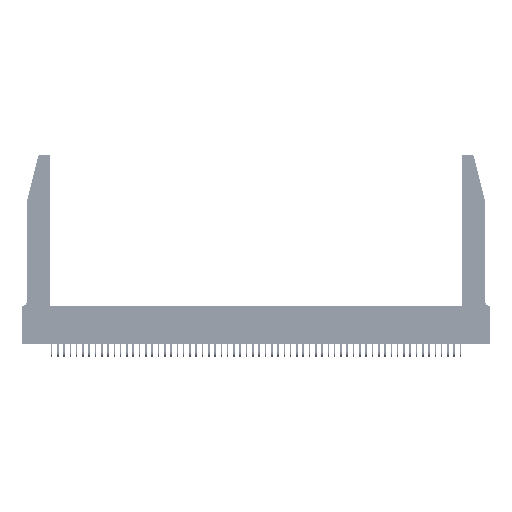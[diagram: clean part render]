
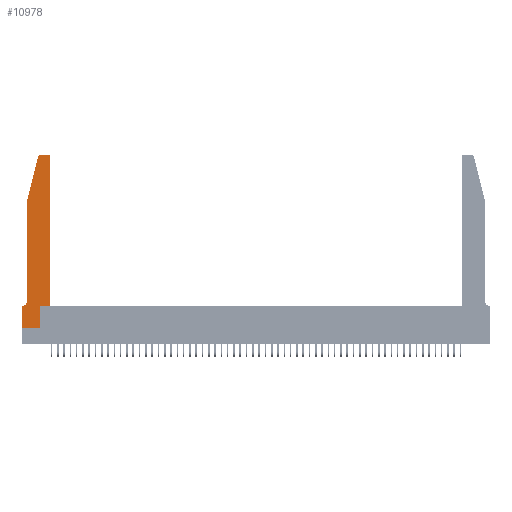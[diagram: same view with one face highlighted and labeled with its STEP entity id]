
A CAD part, top view. The second image highlights one B-rep face of the part: STEP entity #10978.
In plain terms, the highlighted planar face has unit normal (0, 0, 1).
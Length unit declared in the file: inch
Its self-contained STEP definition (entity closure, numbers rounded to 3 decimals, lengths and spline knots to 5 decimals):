
#1144 = EDGE_CURVE ( 'NONE', #27276, #46740, #19152, .T. ) ;
#1185 = ORIENTED_EDGE ( 'NONE', *, *, #3137, .T. ) ;
#1265 = CARTESIAN_POINT ( 'NONE',  ( 0.4505, 0.35, 0.37 ) ) ;
#1358 = ORIENTED_EDGE ( 'NONE', *, *, #42445, .T. ) ;
#1390 = VECTOR ( 'NONE', #35444, 39.37008 ) ;
#2430 = ORIENTED_EDGE ( 'NONE', *, *, #13091, .T. ) ;
#2660 = EDGE_CURVE ( 'NONE', #15259, #50603, #51960, .T. ) ;
#2677 = ORIENTED_EDGE ( 'NONE', *, *, #2660, .T. ) ;
#2962 = CARTESIAN_POINT ( 'NONE',  ( 0.2605, 2.75, 0.37 ) ) ;
#3137 = EDGE_CURVE ( 'NONE', #53790, #24854, #18341, .T. ) ;
#3493 = AXIS2_PLACEMENT_3D ( 'NONE', #33217, #7725, #37428 ) ;
#3852 = VERTEX_POINT ( 'NONE', #5821 ) ;
#4472 = LINE ( 'NONE', #11216, #25912 ) ;
#5068 = CARTESIAN_POINT ( 'NONE',  ( 0.0755, 0.42, 0.37 ) ) ;
#5821 = CARTESIAN_POINT ( 'NONE',  ( 0.4205, 2.75, 0.37 ) ) ;
#5848 = DIRECTION ( 'NONE',  ( 0., 0., 1. ) ) ;
#5897 = ORIENTED_EDGE ( 'NONE', *, *, #17350, .T. ) ;
#6249 = CARTESIAN_POINT ( 'NONE',  ( 0.4505, 2.72, 0.37 ) ) ;
#6460 = CARTESIAN_POINT ( 'NONE',  ( 0., 0., 0.37 ) ) ;
#6992 = ORIENTED_EDGE ( 'NONE', *, *, #1144, .T. ) ;
#7110 = AXIS2_PLACEMENT_3D ( 'NONE', #21053, #42389, #17166 ) ;
#7152 = LINE ( 'NONE', #9784, #39676 ) ;
#7649 = ORIENTED_EDGE ( 'NONE', *, *, #35547, .T. ) ;
#7725 = DIRECTION ( 'NONE',  ( 0., 0., 1. ) ) ;
#9075 = VECTOR ( 'NONE', #31203, 39.37008 ) ;
#9408 = VECTOR ( 'NONE', #23684, 39.37008 ) ;
#9784 = CARTESIAN_POINT ( 'NONE',  ( 0.2865, 0.35, 0.37 ) ) ;
#10311 = ORIENTED_EDGE ( 'NONE', *, *, #40543, .T. ) ;
#10978 = ADVANCED_FACE ( 'NONE', ( #45802 ), #33964, .T. ) ;
#11152 = DIRECTION ( 'NONE',  ( -0.239, -0.971, 0. ) ) ;
#11216 = CARTESIAN_POINT ( 'NONE',  ( 0.4505, 0.35, 0.37 ) ) ;
#11679 = ORIENTED_EDGE ( 'NONE', *, *, #34342, .T. ) ;
#11734 = CARTESIAN_POINT ( 'NONE',  ( 0.4505, 0.35, 0.37 ) ) ;
#11985 = CARTESIAN_POINT ( 'NONE',  ( 0.0755, 2., 0.37 ) ) ;
#12399 = LINE ( 'NONE', #2962, #32286 ) ;
#13091 = EDGE_CURVE ( 'NONE', #15248, #53790, #17243, .T. ) ;
#13307 = AXIS2_PLACEMENT_3D ( 'NONE', #31402, #5848, #35607 ) ;
#13416 = EDGE_CURVE ( 'NONE', #46740, #3852, #35022, .T. ) ;
#13746 = EDGE_CURVE ( 'NONE', #28227, #54357, #7152, .T. ) ;
#14112 = DIRECTION ( 'NONE',  ( 0., 1., 0. ) ) ;
#14314 = VECTOR ( 'NONE', #23885, 39.37008 ) ;
#14790 = CARTESIAN_POINT ( 'NONE',  ( 0., 0., 0.37 ) ) ;
#15248 = VERTEX_POINT ( 'NONE', #41295 ) ;
#15259 = VERTEX_POINT ( 'NONE', #28797 ) ;
#16382 = ORIENTED_EDGE ( 'NONE', *, *, #13416, .T. ) ;
#17166 = DIRECTION ( 'NONE',  ( 1., 0., 0. ) ) ;
#17221 = ORIENTED_EDGE ( 'NONE', *, *, #13746, .T. ) ;
#17243 = CIRCLE ( 'NONE', #13307, 0.03 ) ;
#17350 = EDGE_CURVE ( 'NONE', #37437, #15259, #20083, .T. ) ;
#18341 = LINE ( 'NONE', #36526, #29586 ) ;
#18676 = CARTESIAN_POINT ( 'NONE',  ( 0., 0., 0.37 ) ) ;
#19152 = LINE ( 'NONE', #1265, #9075 ) ;
#20083 = CIRCLE ( 'NONE', #52610, 0.07 ) ;
#20294 = LINE ( 'NONE', #18676, #1390 ) ;
#20798 = LINE ( 'NONE', #6460, #9408 ) ;
#20909 = CARTESIAN_POINT ( 'NONE',  ( 0.0755, 0.35, 0.37 ) ) ;
#21053 = CARTESIAN_POINT ( 'NONE',  ( 0., 0.35, 0.37 ) ) ;
#21184 = EDGE_CURVE ( 'NONE', #50603, #50009, #20294, .T. ) ;
#21426 = CARTESIAN_POINT ( 'NONE',  ( 0.0055, 0.42, 0.37 ) ) ;
#23684 = DIRECTION ( 'NONE',  ( 1., 0., 0. ) ) ;
#23885 = DIRECTION ( 'NONE',  ( 0., -1., 0. ) ) ;
#24854 = VERTEX_POINT ( 'NONE', #11985 ) ;
#25166 = DIRECTION ( 'NONE',  ( -1., 0., 0. ) ) ;
#25652 = DIRECTION ( 'NONE',  ( -1., 0., 0. ) ) ;
#25912 = VECTOR ( 'NONE', #49040, 39.37008 ) ;
#27276 = VERTEX_POINT ( 'NONE', #11734 ) ;
#28227 = VERTEX_POINT ( 'NONE', #29233 ) ;
#28797 = CARTESIAN_POINT ( 'NONE',  ( 0.0055, 0.35, 0.37 ) ) ;
#29233 = CARTESIAN_POINT ( 'NONE',  ( 0.2865, 0., 0.37 ) ) ;
#29586 = VECTOR ( 'NONE', #11152, 39.37008 ) ;
#31203 = DIRECTION ( 'NONE',  ( 0., 1., 0. ) ) ;
#31402 = CARTESIAN_POINT ( 'NONE',  ( 0.284, 2.72, 0.37 ) ) ;
#32286 = VECTOR ( 'NONE', #41272, 39.37008 ) ;
#33217 = CARTESIAN_POINT ( 'NONE',  ( 0.4205, 2.72, 0.37 ) ) ;
#33379 = CARTESIAN_POINT ( 'NONE',  ( 0.25487, 2.72718, 0.37 ) ) ;
#33964 = PLANE ( 'NONE',  #7110 ) ;
#34342 = EDGE_CURVE ( 'NONE', #3852, #15248, #12399, .T. ) ;
#35022 = CIRCLE ( 'NONE', #3493, 0.03 ) ;
#35198 = ORIENTED_EDGE ( 'NONE', *, *, #21184, .T. ) ;
#35444 = DIRECTION ( 'NONE',  ( 0., -1., 0. ) ) ;
#35547 = EDGE_CURVE ( 'NONE', #54357, #27276, #4472, .T. ) ;
#35607 = DIRECTION ( 'NONE',  ( 1., 0., 0. ) ) ;
#36526 = CARTESIAN_POINT ( 'NONE',  ( 0.0755, 2., 0.37 ) ) ;
#36805 = LINE ( 'NONE', #40624, #14314 ) ;
#37428 = DIRECTION ( 'NONE',  ( 1., 0., 0. ) ) ;
#37437 = VERTEX_POINT ( 'NONE', #5068 ) ;
#39676 = VECTOR ( 'NONE', #14112, 39.37008 ) ;
#40543 = EDGE_CURVE ( 'NONE', #50009, #28227, #20798, .T. ) ;
#40624 = CARTESIAN_POINT ( 'NONE',  ( 0.0755, 2., 0.37 ) ) ;
#41272 = DIRECTION ( 'NONE',  ( -1., 0., 0. ) ) ;
#41295 = CARTESIAN_POINT ( 'NONE',  ( 0.284, 2.75, 0.37 ) ) ;
#42389 = DIRECTION ( 'NONE',  ( 0., 0., 1. ) ) ;
#42445 = EDGE_CURVE ( 'NONE', #24854, #37437, #36805, .T. ) ;
#45802 = FACE_OUTER_BOUND ( 'NONE', #51962, .T. ) ;
#46740 = VERTEX_POINT ( 'NONE', #6249 ) ;
#49040 = DIRECTION ( 'NONE',  ( 1., 0., 0. ) ) ;
#49807 = CARTESIAN_POINT ( 'NONE',  ( 0.2865, 0.35, 0.37 ) ) ;
#50009 = VERTEX_POINT ( 'NONE', #14790 ) ;
#50603 = VERTEX_POINT ( 'NONE', #52294 ) ;
#50617 = VECTOR ( 'NONE', #25166, 39.37008 ) ;
#50803 = DIRECTION ( 'NONE',  ( 0., 0., -1. ) ) ;
#51960 = LINE ( 'NONE', #20909, #50617 ) ;
#51962 = EDGE_LOOP ( 'NONE', ( #11679, #2430, #1185, #1358, #5897, #2677, #35198, #10311, #17221, #7649, #6992, #16382 ) ) ;
#52294 = CARTESIAN_POINT ( 'NONE',  ( 0., 0.35, 0.37 ) ) ;
#52610 = AXIS2_PLACEMENT_3D ( 'NONE', #21426, #50803, #25652 ) ;
#53790 = VERTEX_POINT ( 'NONE', #33379 ) ;
#54357 = VERTEX_POINT ( 'NONE', #49807 ) ;
